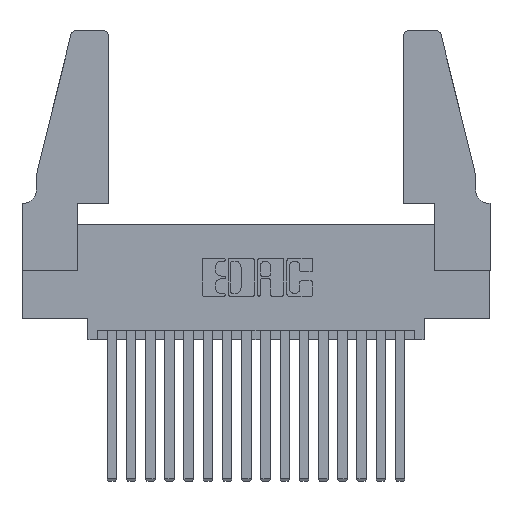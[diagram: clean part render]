
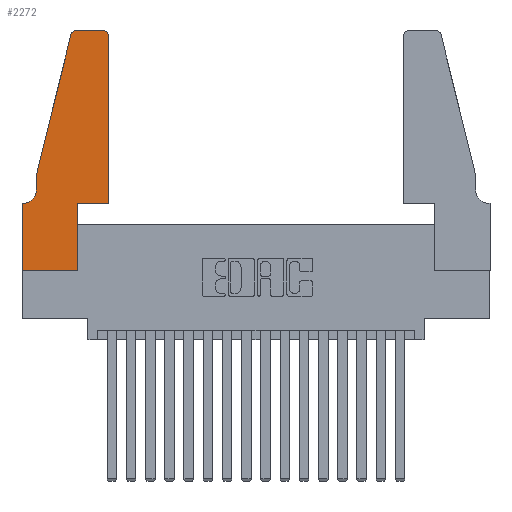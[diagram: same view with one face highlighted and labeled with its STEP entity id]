
A CAD part, top view. The second image highlights one B-rep face of the part: STEP entity #2272.
In plain terms, the highlighted planar face has unit normal (0, 0, 1).
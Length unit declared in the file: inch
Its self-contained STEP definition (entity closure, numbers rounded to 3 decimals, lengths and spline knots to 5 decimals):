
#6 = VERTEX_POINT ( 'NONE', #3235 ) ;
#267 = DIRECTION ( 'NONE',  ( 1., 0., 0. ) ) ;
#580 = EDGE_CURVE ( 'NONE', #2121, #15309, #1678, .T. ) ;
#636 = CIRCLE ( 'NONE', #8554, 0.03 ) ;
#990 = DIRECTION ( 'NONE',  ( 1., 0., 0. ) ) ;
#1042 = VECTOR ( 'NONE', #18035, 39.37008 ) ;
#1319 = LINE ( 'NONE', #17727, #15368 ) ;
#1376 = CARTESIAN_POINT ( 'NONE',  ( 0.2865, 0.35, 0.37 ) ) ;
#1455 = EDGE_CURVE ( 'NONE', #15783, #14819, #16893, .T. ) ;
#1531 = VECTOR ( 'NONE', #17676, 39.37008 ) ;
#1626 = VERTEX_POINT ( 'NONE', #5460 ) ;
#1635 = DIRECTION ( 'NONE',  ( 0., 0., 1. ) ) ;
#1651 = AXIS2_PLACEMENT_3D ( 'NONE', #12941, #8613, #14118 ) ;
#1678 = LINE ( 'NONE', #4156, #1042 ) ;
#2121 = VERTEX_POINT ( 'NONE', #12323 ) ;
#2272 = ADVANCED_FACE ( 'NONE', ( #7893 ), #15188, .T. ) ;
#2400 = EDGE_CURVE ( 'NONE', #14237, #6, #3714, .T. ) ;
#2752 = ORIENTED_EDGE ( 'NONE', *, *, #12537, .T. ) ;
#2840 = LINE ( 'NONE', #14300, #6534 ) ;
#3235 = CARTESIAN_POINT ( 'NONE',  ( 0.4505, 0.35, 0.37 ) ) ;
#3407 = EDGE_LOOP ( 'NONE', ( #9178, #6394, #6463, #17206, #2752, #16685, #10479, #17366, #14558, #13321, #15251, #8767 ) ) ;
#3714 = LINE ( 'NONE', #13374, #8112 ) ;
#3760 = LINE ( 'NONE', #7976, #1531 ) ;
#4156 = CARTESIAN_POINT ( 'NONE',  ( 0.0755, 0.5, 0.37 ) ) ;
#5460 = CARTESIAN_POINT ( 'NONE',  ( 0.4505, 1.22, 0.37 ) ) ;
#5747 = VECTOR ( 'NONE', #18174, 39.37008 ) ;
#5831 = DIRECTION ( 'NONE',  ( 1., 0., 0. ) ) ;
#5907 = CARTESIAN_POINT ( 'NONE',  ( 0.4205, 1.22, 0.37 ) ) ;
#6203 = CARTESIAN_POINT ( 'NONE',  ( 0.0755, 0.5, 0.37 ) ) ;
#6394 = ORIENTED_EDGE ( 'NONE', *, *, #8426, .T. ) ;
#6463 = ORIENTED_EDGE ( 'NONE', *, *, #580, .T. ) ;
#6512 = VECTOR ( 'NONE', #5831, 39.37008 ) ;
#6534 = VECTOR ( 'NONE', #10141, 39.37008 ) ;
#6623 = EDGE_CURVE ( 'NONE', #1626, #11709, #7515, .T. ) ;
#6697 = VERTEX_POINT ( 'NONE', #15542 ) ;
#6883 = CARTESIAN_POINT ( 'NONE',  ( 0.2605, 1.25, 0.37 ) ) ;
#7081 = AXIS2_PLACEMENT_3D ( 'NONE', #12484, #9495, #13849 ) ;
#7087 = EDGE_CURVE ( 'NONE', #6, #1626, #2840, .T. ) ;
#7125 = DIRECTION ( 'NONE',  ( -1., 0., 0. ) ) ;
#7164 = EDGE_CURVE ( 'NONE', #14819, #6697, #15805, .T. ) ;
#7354 = CARTESIAN_POINT ( 'NONE',  ( 0., 0., 0.37 ) ) ;
#7515 = CIRCLE ( 'NONE', #14721, 0.03 ) ;
#7882 = CARTESIAN_POINT ( 'NONE',  ( 0.0755, 0.42, 0.37 ) ) ;
#7893 = FACE_OUTER_BOUND ( 'NONE', #3407, .T. ) ;
#7976 = CARTESIAN_POINT ( 'NONE',  ( 0.2865, 0.35, 0.37 ) ) ;
#8112 = VECTOR ( 'NONE', #12461, 39.37008 ) ;
#8217 = CARTESIAN_POINT ( 'NONE',  ( 0.0055, 0.35, 0.37 ) ) ;
#8398 = CARTESIAN_POINT ( 'NONE',  ( 0., 0., 0.37 ) ) ;
#8426 = EDGE_CURVE ( 'NONE', #13267, #2121, #636, .T. ) ;
#8554 = AXIS2_PLACEMENT_3D ( 'NONE', #9481, #11588, #990 ) ;
#8602 = LINE ( 'NONE', #6203, #14706 ) ;
#8613 = DIRECTION ( 'NONE',  ( 0., 0., -1. ) ) ;
#8725 = CARTESIAN_POINT ( 'NONE',  ( 0., 0.35, 0.37 ) ) ;
#8767 = ORIENTED_EDGE ( 'NONE', *, *, #6623, .T. ) ;
#8800 = EDGE_CURVE ( 'NONE', #6697, #14237, #3760, .T. ) ;
#8926 = EDGE_CURVE ( 'NONE', #11709, #13267, #11858, .T. ) ;
#9064 = EDGE_CURVE ( 'NONE', #15309, #14723, #8602, .T. ) ;
#9119 = CIRCLE ( 'NONE', #1651, 0.07 ) ;
#9178 = ORIENTED_EDGE ( 'NONE', *, *, #8926, .T. ) ;
#9187 = CARTESIAN_POINT ( 'NONE',  ( 0.0755, 0.5, 0.37 ) ) ;
#9481 = CARTESIAN_POINT ( 'NONE',  ( 0.284, 1.22, 0.37 ) ) ;
#9495 = DIRECTION ( 'NONE',  ( 0., 0., 1. ) ) ;
#9611 = EDGE_CURVE ( 'NONE', #14277, #15783, #1319, .T. ) ;
#10141 = DIRECTION ( 'NONE',  ( 0., 1., 0. ) ) ;
#10472 = CARTESIAN_POINT ( 'NONE',  ( 0.284, 1.25, 0.37 ) ) ;
#10479 = ORIENTED_EDGE ( 'NONE', *, *, #1455, .T. ) ;
#11482 = DIRECTION ( 'NONE',  ( -1., 0., 0. ) ) ;
#11588 = DIRECTION ( 'NONE',  ( 0., 0., 1. ) ) ;
#11709 = VERTEX_POINT ( 'NONE', #12540 ) ;
#11858 = LINE ( 'NONE', #6883, #14271 ) ;
#12323 = CARTESIAN_POINT ( 'NONE',  ( 0.25487, 1.22718, 0.37 ) ) ;
#12461 = DIRECTION ( 'NONE',  ( 1., 0., 0. ) ) ;
#12484 = CARTESIAN_POINT ( 'NONE',  ( 0., 0.35, 0.37 ) ) ;
#12537 = EDGE_CURVE ( 'NONE', #14723, #14277, #9119, .T. ) ;
#12540 = CARTESIAN_POINT ( 'NONE',  ( 0.4205, 1.25, 0.37 ) ) ;
#12941 = CARTESIAN_POINT ( 'NONE',  ( 0.0055, 0.42, 0.37 ) ) ;
#13267 = VERTEX_POINT ( 'NONE', #10472 ) ;
#13321 = ORIENTED_EDGE ( 'NONE', *, *, #2400, .T. ) ;
#13374 = CARTESIAN_POINT ( 'NONE',  ( 0.4505, 0.35, 0.37 ) ) ;
#13849 = DIRECTION ( 'NONE',  ( 1., 0., 0. ) ) ;
#14118 = DIRECTION ( 'NONE',  ( -1., 0., 0. ) ) ;
#14237 = VERTEX_POINT ( 'NONE', #1376 ) ;
#14271 = VECTOR ( 'NONE', #7125, 39.37008 ) ;
#14277 = VERTEX_POINT ( 'NONE', #8217 ) ;
#14300 = CARTESIAN_POINT ( 'NONE',  ( 0.4505, 0.35, 0.37 ) ) ;
#14558 = ORIENTED_EDGE ( 'NONE', *, *, #8800, .T. ) ;
#14706 = VECTOR ( 'NONE', #15974, 39.37008 ) ;
#14721 = AXIS2_PLACEMENT_3D ( 'NONE', #5907, #1635, #267 ) ;
#14723 = VERTEX_POINT ( 'NONE', #7882 ) ;
#14819 = VERTEX_POINT ( 'NONE', #15036 ) ;
#15036 = CARTESIAN_POINT ( 'NONE',  ( 0., 0., 0.37 ) ) ;
#15188 = PLANE ( 'NONE',  #7081 ) ;
#15251 = ORIENTED_EDGE ( 'NONE', *, *, #7087, .T. ) ;
#15309 = VERTEX_POINT ( 'NONE', #9187 ) ;
#15368 = VECTOR ( 'NONE', #11482, 39.37008 ) ;
#15542 = CARTESIAN_POINT ( 'NONE',  ( 0.2865, 0., 0.37 ) ) ;
#15783 = VERTEX_POINT ( 'NONE', #8725 ) ;
#15805 = LINE ( 'NONE', #7354, #6512 ) ;
#15974 = DIRECTION ( 'NONE',  ( 0., -1., 0. ) ) ;
#16685 = ORIENTED_EDGE ( 'NONE', *, *, #9611, .T. ) ;
#16893 = LINE ( 'NONE', #8398, #5747 ) ;
#17206 = ORIENTED_EDGE ( 'NONE', *, *, #9064, .T. ) ;
#17366 = ORIENTED_EDGE ( 'NONE', *, *, #7164, .T. ) ;
#17676 = DIRECTION ( 'NONE',  ( 0., 1., 0. ) ) ;
#17727 = CARTESIAN_POINT ( 'NONE',  ( 0.0755, 0.35, 0.37 ) ) ;
#18035 = DIRECTION ( 'NONE',  ( -0.239, -0.971, 0. ) ) ;
#18174 = DIRECTION ( 'NONE',  ( 0., -1., 0. ) ) ;
